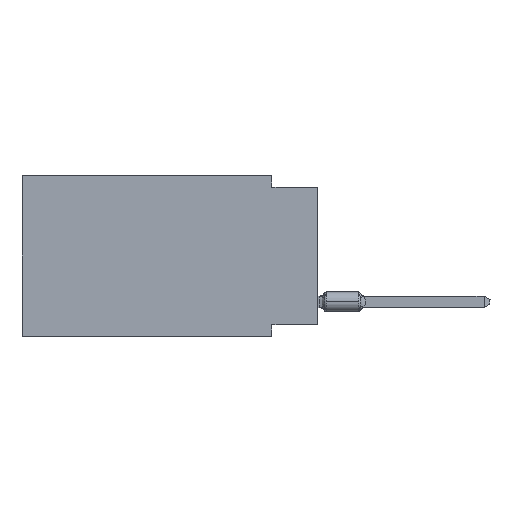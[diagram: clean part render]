
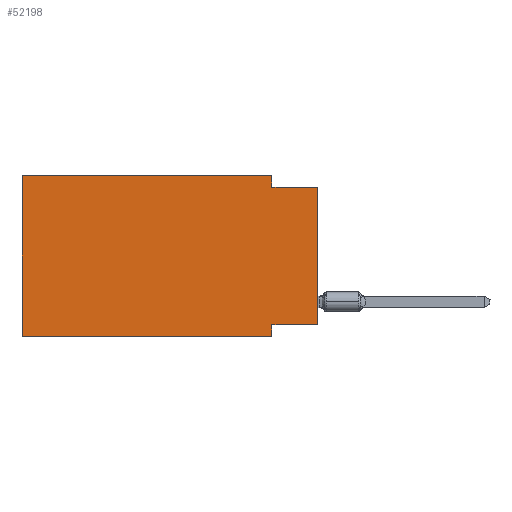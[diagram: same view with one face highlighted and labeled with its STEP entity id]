
A CAD part, left-side view. The second image highlights one B-rep face of the part: STEP entity #52198.
In plain terms, the highlighted planar face has unit normal (-1, 0, 0).
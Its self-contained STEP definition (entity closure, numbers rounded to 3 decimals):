
#239 = DIRECTION ( 'NONE',  ( 1., 0., 0. ) ) ;
#473 = LINE ( 'NONE', #38837, #52331 ) ;
#2230 = VERTEX_POINT ( 'NONE', #18253 ) ;
#3408 = CARTESIAN_POINT ( 'NONE',  ( 0., 16.383, -8.89 ) ) ;
#5126 = VECTOR ( 'NONE', #18871, 1000. ) ;
#5150 = CARTESIAN_POINT ( 'NONE',  ( 0., 0., -0.635 ) ) ;
#6033 = LINE ( 'NONE', #26334, #54024 ) ;
#6189 = AXIS2_PLACEMENT_3D ( 'NONE', #12582, #239, #12305 ) ;
#6679 = DIRECTION ( 'NONE',  ( 0., 0., -1. ) ) ;
#7343 = EDGE_CURVE ( 'NONE', #24415, #18816, #6033, .T. ) ;
#8201 = FACE_OUTER_BOUND ( 'NONE', #19201, .T. ) ;
#8356 = ORIENTED_EDGE ( 'NONE', *, *, #43549, .F. ) ;
#9291 = VECTOR ( 'NONE', #47134, 1000. ) ;
#9794 = DIRECTION ( 'NONE',  ( 0., -1., 0. ) ) ;
#10529 = VERTEX_POINT ( 'NONE', #28828 ) ;
#10714 = ORIENTED_EDGE ( 'NONE', *, *, #19431, .F. ) ;
#12305 = DIRECTION ( 'NONE',  ( 0., 0., -1. ) ) ;
#12582 = CARTESIAN_POINT ( 'NONE',  ( 0., 16.383, 0. ) ) ;
#13465 = EDGE_CURVE ( 'NONE', #33885, #17337, #25671, .T. ) ;
#13935 = LINE ( 'NONE', #18322, #9291 ) ;
#15117 = EDGE_CURVE ( 'NONE', #18816, #17337, #473, .T. ) ;
#15335 = CARTESIAN_POINT ( 'NONE',  ( 0., 16.383, 0. ) ) ;
#15378 = VECTOR ( 'NONE', #42377, 1000. ) ;
#17337 = VERTEX_POINT ( 'NONE', #5150 ) ;
#18253 = CARTESIAN_POINT ( 'NONE',  ( 0., 2.54, -8.89 ) ) ;
#18322 = CARTESIAN_POINT ( 'NONE',  ( 0., 0., -8.255 ) ) ;
#18816 = VERTEX_POINT ( 'NONE', #24529 ) ;
#18871 = DIRECTION ( 'NONE',  ( 0., 0., 1. ) ) ;
#19201 = EDGE_LOOP ( 'NONE', ( #32353, #25296, #20491, #10714, #43824, #46906, #39270, #8356 ) ) ;
#19431 = EDGE_CURVE ( 'NONE', #10529, #24415, #35370, .T. ) ;
#20491 = ORIENTED_EDGE ( 'NONE', *, *, #7343, .F. ) ;
#21542 = CARTESIAN_POINT ( 'NONE',  ( 0., 0., 0. ) ) ;
#24415 = VERTEX_POINT ( 'NONE', #39139 ) ;
#24529 = CARTESIAN_POINT ( 'NONE',  ( 0., 2.54, -0.635 ) ) ;
#25296 = ORIENTED_EDGE ( 'NONE', *, *, #15117, .F. ) ;
#25671 = LINE ( 'NONE', #21542, #15378 ) ;
#26305 = CARTESIAN_POINT ( 'NONE',  ( 0., 2.54, -8.255 ) ) ;
#26334 = CARTESIAN_POINT ( 'NONE',  ( 0., 2.54, 0. ) ) ;
#27517 = LINE ( 'NONE', #35459, #47523 ) ;
#28438 = EDGE_CURVE ( 'NONE', #43031, #2230, #54096, .T. ) ;
#28828 = CARTESIAN_POINT ( 'NONE',  ( 0., 16.383, 0. ) ) ;
#32028 = LINE ( 'NONE', #47947, #5126 ) ;
#32353 = ORIENTED_EDGE ( 'NONE', *, *, #13465, .T. ) ;
#32597 = PLANE ( 'NONE',  #6189 ) ;
#32676 = CARTESIAN_POINT ( 'NONE',  ( 0., 16.383, -8.89 ) ) ;
#33885 = VERTEX_POINT ( 'NONE', #54196 ) ;
#35076 = DIRECTION ( 'NONE',  ( 0., 0., -1. ) ) ;
#35370 = LINE ( 'NONE', #15335, #36253 ) ;
#35459 = CARTESIAN_POINT ( 'NONE',  ( 0., 2.54, -8.89 ) ) ;
#36253 = VECTOR ( 'NONE', #48248, 1000. ) ;
#37644 = DIRECTION ( 'NONE',  ( 0., -1., 0. ) ) ;
#38837 = CARTESIAN_POINT ( 'NONE',  ( 0., 0., -0.635 ) ) ;
#39139 = CARTESIAN_POINT ( 'NONE',  ( 0., 2.54, 0. ) ) ;
#39205 = EDGE_CURVE ( 'NONE', #43031, #10529, #32028, .T. ) ;
#39270 = ORIENTED_EDGE ( 'NONE', *, *, #48399, .F. ) ;
#42377 = DIRECTION ( 'NONE',  ( 0., 0., 1. ) ) ;
#42406 = VECTOR ( 'NONE', #37644, 1000. ) ;
#43031 = VERTEX_POINT ( 'NONE', #32676 ) ;
#43549 = EDGE_CURVE ( 'NONE', #33885, #44408, #13935, .T. ) ;
#43824 = ORIENTED_EDGE ( 'NONE', *, *, #39205, .F. ) ;
#44408 = VERTEX_POINT ( 'NONE', #26305 ) ;
#46906 = ORIENTED_EDGE ( 'NONE', *, *, #28438, .T. ) ;
#47134 = DIRECTION ( 'NONE',  ( 0., 1., 0. ) ) ;
#47523 = VECTOR ( 'NONE', #6679, 1000. ) ;
#47947 = CARTESIAN_POINT ( 'NONE',  ( 0., 16.383, 0. ) ) ;
#48248 = DIRECTION ( 'NONE',  ( 0., -1., 0. ) ) ;
#48399 = EDGE_CURVE ( 'NONE', #44408, #2230, #27517, .T. ) ;
#52198 = ADVANCED_FACE ( 'NONE', ( #8201 ), #32597, .F. ) ;
#52331 = VECTOR ( 'NONE', #9794, 1000. ) ;
#54024 = VECTOR ( 'NONE', #35076, 1000. ) ;
#54096 = LINE ( 'NONE', #3408, #42406 ) ;
#54196 = CARTESIAN_POINT ( 'NONE',  ( 0., 0., -8.255 ) ) ;
